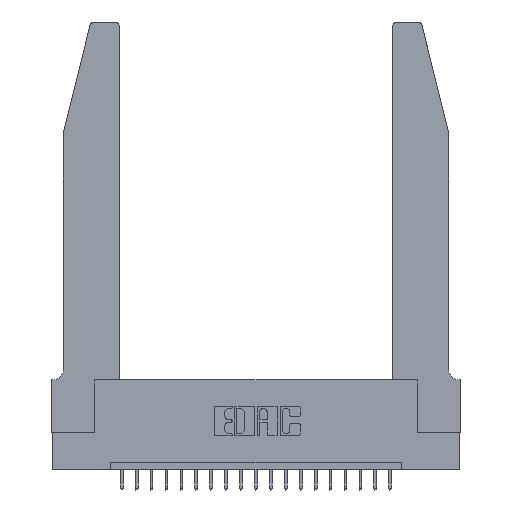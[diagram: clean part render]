
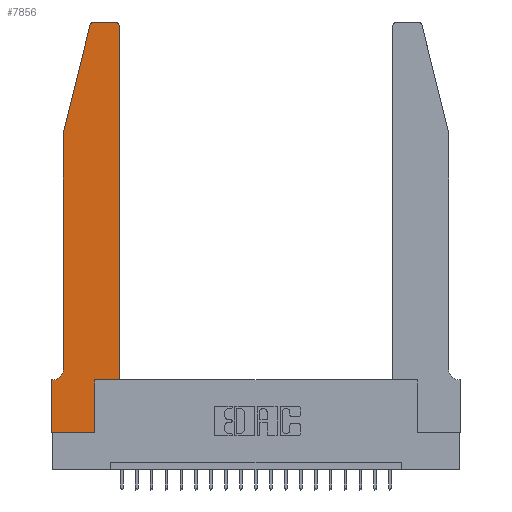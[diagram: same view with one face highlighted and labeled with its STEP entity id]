
A CAD part, top view. The second image highlights one B-rep face of the part: STEP entity #7856.
In plain terms, the highlighted planar face has unit normal (0, 0, 1).
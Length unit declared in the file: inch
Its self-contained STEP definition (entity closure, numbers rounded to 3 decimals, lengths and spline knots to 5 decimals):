
#238 = DIRECTION ( 'NONE',  ( 0., 0., -1. ) ) ;
#436 = CARTESIAN_POINT ( 'NONE',  ( 0.4205, 2.72, 0.37 ) ) ;
#441 = ORIENTED_EDGE ( 'NONE', *, *, #18980, .T. ) ;
#698 = CARTESIAN_POINT ( 'NONE',  ( 0.284, 2.72, 0.37 ) ) ;
#924 = VERTEX_POINT ( 'NONE', #3249 ) ;
#995 = CARTESIAN_POINT ( 'NONE',  ( 0.2865, 0.35, 0.37 ) ) ;
#2189 = CARTESIAN_POINT ( 'NONE',  ( 0.4505, 0.35, 0.37 ) ) ;
#2391 = DIRECTION ( 'NONE',  ( 0., 0., 1. ) ) ;
#2572 = ORIENTED_EDGE ( 'NONE', *, *, #4061, .T. ) ;
#2729 = EDGE_CURVE ( 'NONE', #3832, #14829, #5360, .T. ) ;
#2811 = DIRECTION ( 'NONE',  ( -0.239, -0.971, 0. ) ) ;
#2847 = AXIS2_PLACEMENT_3D ( 'NONE', #12090, #238, #13979 ) ;
#3249 = CARTESIAN_POINT ( 'NONE',  ( 0.2865, 0.35, 0.37 ) ) ;
#3556 = AXIS2_PLACEMENT_3D ( 'NONE', #698, #2391, #14223 ) ;
#3557 = DIRECTION ( 'NONE',  ( -1., 0., 0. ) ) ;
#3630 = CARTESIAN_POINT ( 'NONE',  ( 0.4505, 0.35, 0.37 ) ) ;
#3724 = ORIENTED_EDGE ( 'NONE', *, *, #17536, .T. ) ;
#3777 = DIRECTION ( 'NONE',  ( 1., 0., 0. ) ) ;
#3832 = VERTEX_POINT ( 'NONE', #10590 ) ;
#4061 = EDGE_CURVE ( 'NONE', #15766, #12209, #4667, .T. ) ;
#4223 = VERTEX_POINT ( 'NONE', #14040 ) ;
#4667 = CIRCLE ( 'NONE', #10100, 0.03 ) ;
#5191 = CARTESIAN_POINT ( 'NONE',  ( 0.25487, 2.72718, 0.37 ) ) ;
#5332 = CARTESIAN_POINT ( 'NONE',  ( 0., 0., 0.37 ) ) ;
#5360 = LINE ( 'NONE', #10661, #8295 ) ;
#6240 = VERTEX_POINT ( 'NONE', #8837 ) ;
#6472 = DIRECTION ( 'NONE',  ( 0., 0., 1. ) ) ;
#6480 = CARTESIAN_POINT ( 'NONE',  ( 0.0755, 2., 0.37 ) ) ;
#6603 = EDGE_CURVE ( 'NONE', #12209, #12999, #8697, .T. ) ;
#7027 = LINE ( 'NONE', #5332, #14321 ) ;
#7326 = DIRECTION ( 'NONE',  ( 0., 0., 1. ) ) ;
#7451 = EDGE_CURVE ( 'NONE', #14829, #4223, #7027, .T. ) ;
#7781 = LINE ( 'NONE', #995, #12082 ) ;
#7856 = ADVANCED_FACE ( 'NONE', ( #14250 ), #19507, .T. ) ;
#8190 = EDGE_CURVE ( 'NONE', #12999, #15464, #20067, .T. ) ;
#8216 = ORIENTED_EDGE ( 'NONE', *, *, #8190, .T. ) ;
#8295 = VECTOR ( 'NONE', #3557, 39.37008 ) ;
#8459 = EDGE_CURVE ( 'NONE', #16656, #3832, #20082, .T. ) ;
#8591 = CARTESIAN_POINT ( 'NONE',  ( 0.2605, 2.75, 0.37 ) ) ;
#8595 = AXIS2_PLACEMENT_3D ( 'NONE', #16361, #6472, #9869 ) ;
#8697 = LINE ( 'NONE', #8591, #14627 ) ;
#8837 = CARTESIAN_POINT ( 'NONE',  ( 0.0755, 2., 0.37 ) ) ;
#9502 = VERTEX_POINT ( 'NONE', #15547 ) ;
#9808 = DIRECTION ( 'NONE',  ( 0., 1., 0. ) ) ;
#9869 = DIRECTION ( 'NONE',  ( 1., 0., 0. ) ) ;
#10100 = AXIS2_PLACEMENT_3D ( 'NONE', #436, #7326, #21016 ) ;
#10116 = LINE ( 'NONE', #21891, #19948 ) ;
#10590 = CARTESIAN_POINT ( 'NONE',  ( 0.0055, 0.35, 0.37 ) ) ;
#10627 = EDGE_CURVE ( 'NONE', #6240, #16656, #21870, .T. ) ;
#10661 = CARTESIAN_POINT ( 'NONE',  ( 0.0755, 0.35, 0.37 ) ) ;
#10960 = ORIENTED_EDGE ( 'NONE', *, *, #2729, .T. ) ;
#10977 = VECTOR ( 'NONE', #21298, 39.37008 ) ;
#11024 = ORIENTED_EDGE ( 'NONE', *, *, #7451, .T. ) ;
#11496 = CARTESIAN_POINT ( 'NONE',  ( 0.0755, 2., 0.37 ) ) ;
#12082 = VECTOR ( 'NONE', #9808, 39.37008 ) ;
#12090 = CARTESIAN_POINT ( 'NONE',  ( 0.0055, 0.42, 0.37 ) ) ;
#12209 = VERTEX_POINT ( 'NONE', #13292 ) ;
#12795 = VECTOR ( 'NONE', #3777, 39.37008 ) ;
#12999 = VERTEX_POINT ( 'NONE', #21621 ) ;
#13249 = VERTEX_POINT ( 'NONE', #3630 ) ;
#13292 = CARTESIAN_POINT ( 'NONE',  ( 0.4205, 2.75, 0.37 ) ) ;
#13979 = DIRECTION ( 'NONE',  ( -1., 0., 0. ) ) ;
#14031 = CARTESIAN_POINT ( 'NONE',  ( 0., 0., 0.37 ) ) ;
#14040 = CARTESIAN_POINT ( 'NONE',  ( 0., 0., 0.37 ) ) ;
#14223 = DIRECTION ( 'NONE',  ( 1., 0., 0. ) ) ;
#14250 = FACE_OUTER_BOUND ( 'NONE', #21071, .T. ) ;
#14321 = VECTOR ( 'NONE', #20511, 39.37008 ) ;
#14502 = CARTESIAN_POINT ( 'NONE',  ( 0.4505, 2.72, 0.37 ) ) ;
#14627 = VECTOR ( 'NONE', #15428, 39.37008 ) ;
#14829 = VERTEX_POINT ( 'NONE', #20698 ) ;
#14888 = ORIENTED_EDGE ( 'NONE', *, *, #16951, .T. ) ;
#15428 = DIRECTION ( 'NONE',  ( -1., 0., 0. ) ) ;
#15464 = VERTEX_POINT ( 'NONE', #5191 ) ;
#15547 = CARTESIAN_POINT ( 'NONE',  ( 0.2865, 0., 0.37 ) ) ;
#15766 = VERTEX_POINT ( 'NONE', #14502 ) ;
#15773 = ORIENTED_EDGE ( 'NONE', *, *, #10627, .T. ) ;
#16001 = EDGE_CURVE ( 'NONE', #924, #13249, #21520, .T. ) ;
#16147 = LINE ( 'NONE', #14031, #12795 ) ;
#16361 = CARTESIAN_POINT ( 'NONE',  ( 0., 0.35, 0.37 ) ) ;
#16656 = VERTEX_POINT ( 'NONE', #17009 ) ;
#16951 = EDGE_CURVE ( 'NONE', #9502, #924, #7781, .T. ) ;
#17009 = CARTESIAN_POINT ( 'NONE',  ( 0.0755, 0.42, 0.37 ) ) ;
#17272 = ORIENTED_EDGE ( 'NONE', *, *, #18347, .T. ) ;
#17425 = VECTOR ( 'NONE', #2811, 39.37008 ) ;
#17536 = EDGE_CURVE ( 'NONE', #13249, #15766, #10116, .T. ) ;
#18168 = DIRECTION ( 'NONE',  ( 0., -1., 0. ) ) ;
#18218 = LINE ( 'NONE', #11496, #17425 ) ;
#18347 = EDGE_CURVE ( 'NONE', #15464, #6240, #18218, .T. ) ;
#18463 = ORIENTED_EDGE ( 'NONE', *, *, #16001, .T. ) ;
#18961 = DIRECTION ( 'NONE',  ( 0., 1., 0. ) ) ;
#18980 = EDGE_CURVE ( 'NONE', #4223, #9502, #16147, .T. ) ;
#19086 = VECTOR ( 'NONE', #18168, 39.37008 ) ;
#19507 = PLANE ( 'NONE',  #8595 ) ;
#19548 = ORIENTED_EDGE ( 'NONE', *, *, #8459, .T. ) ;
#19948 = VECTOR ( 'NONE', #18961, 39.37008 ) ;
#20067 = CIRCLE ( 'NONE', #3556, 0.03 ) ;
#20082 = CIRCLE ( 'NONE', #2847, 0.07 ) ;
#20511 = DIRECTION ( 'NONE',  ( 0., -1., 0. ) ) ;
#20698 = CARTESIAN_POINT ( 'NONE',  ( 0., 0.35, 0.37 ) ) ;
#21016 = DIRECTION ( 'NONE',  ( 1., 0., 0. ) ) ;
#21071 = EDGE_LOOP ( 'NONE', ( #21312, #8216, #17272, #15773, #19548, #10960, #11024, #441, #14888, #18463, #3724, #2572 ) ) ;
#21298 = DIRECTION ( 'NONE',  ( 1., 0., 0. ) ) ;
#21312 = ORIENTED_EDGE ( 'NONE', *, *, #6603, .T. ) ;
#21520 = LINE ( 'NONE', #2189, #10977 ) ;
#21621 = CARTESIAN_POINT ( 'NONE',  ( 0.284, 2.75, 0.37 ) ) ;
#21870 = LINE ( 'NONE', #6480, #19086 ) ;
#21891 = CARTESIAN_POINT ( 'NONE',  ( 0.4505, 0.35, 0.37 ) ) ;
